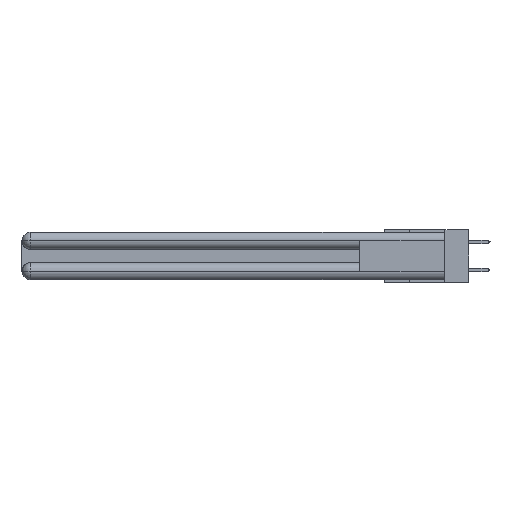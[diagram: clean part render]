
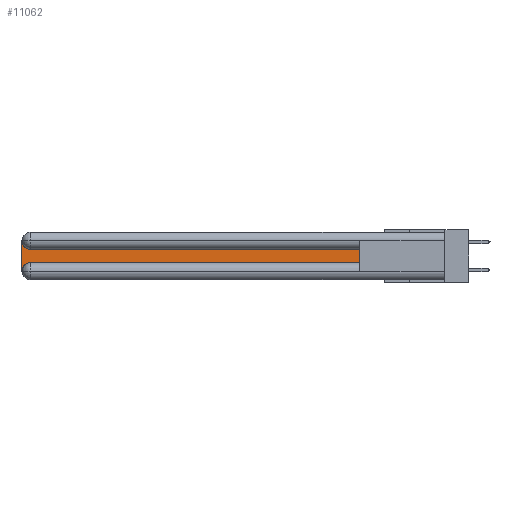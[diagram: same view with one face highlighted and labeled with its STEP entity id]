
A CAD part, left-side view. The second image highlights one B-rep face of the part: STEP entity #11062.
In plain terms, the highlighted planar face has unit normal (-1, 0, 0).
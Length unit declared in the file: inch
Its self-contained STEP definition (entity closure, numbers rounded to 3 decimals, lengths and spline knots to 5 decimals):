
#332 = LINE ( 'NONE', #25507, #10445 ) ;
#1689 = CIRCLE ( 'NONE', #16455, 0.06 ) ;
#1822 = LINE ( 'NONE', #25973, #23637 ) ;
#2093 = DIRECTION ( 'NONE',  ( 0., 0., -1. ) ) ;
#2813 = DIRECTION ( 'NONE',  ( 0., 0., -1. ) ) ;
#4516 = VECTOR ( 'NONE', #6964, 39.37008 ) ;
#6109 = EDGE_CURVE ( 'NONE', #26806, #26462, #1689, .T. ) ;
#6590 = CARTESIAN_POINT ( 'NONE',  ( 0.075, 0.6, -0.1225 ) ) ;
#6612 = EDGE_CURVE ( 'NONE', #22815, #7374, #21521, .T. ) ;
#6964 = DIRECTION ( 'NONE',  ( 0., 1., 0. ) ) ;
#7184 = DIRECTION ( 'NONE',  ( 1., 0., 0. ) ) ;
#7374 = VERTEX_POINT ( 'NONE', #23820 ) ;
#7616 = CARTESIAN_POINT ( 'NONE',  ( 0.075, 3., -0.2175 ) ) ;
#8498 = CARTESIAN_POINT ( 'NONE',  ( 0.075, 2.94, -0.2775 ) ) ;
#8811 = CARTESIAN_POINT ( 'NONE',  ( 0.075, 2.94, -0.0625 ) ) ;
#9150 = EDGE_CURVE ( 'NONE', #18460, #16581, #1822, .T. ) ;
#10445 = VECTOR ( 'NONE', #13276, 39.37008 ) ;
#11062 = ADVANCED_FACE ( 'NONE', ( #26787 ), #11156, .F. ) ;
#11156 = PLANE ( 'NONE',  #26077 ) ;
#12136 = ORIENTED_EDGE ( 'NONE', *, *, #12547, .T. ) ;
#12547 = EDGE_CURVE ( 'NONE', #7374, #18460, #332, .T. ) ;
#12778 = ORIENTED_EDGE ( 'NONE', *, *, #25248, .T. ) ;
#13134 = CARTESIAN_POINT ( 'NONE',  ( 0.075, 0.6, -0.1225 ) ) ;
#13201 = CARTESIAN_POINT ( 'NONE',  ( 0.075, 3., -0.2775 ) ) ;
#13276 = DIRECTION ( 'NONE',  ( 0., -1., 0. ) ) ;
#13728 = EDGE_CURVE ( 'NONE', #16581, #26806, #17598, .T. ) ;
#14617 = DIRECTION ( 'NONE',  ( 1., 0., 0. ) ) ;
#14838 = ORIENTED_EDGE ( 'NONE', *, *, #9150, .T. ) ;
#16455 = AXIS2_PLACEMENT_3D ( 'NONE', #8811, #23503, #23312 ) ;
#16526 = ORIENTED_EDGE ( 'NONE', *, *, #6109, .T. ) ;
#16581 = VERTEX_POINT ( 'NONE', #6590 ) ;
#17197 = ORIENTED_EDGE ( 'NONE', *, *, #13728, .T. ) ;
#17350 = DIRECTION ( 'NONE',  ( 0., 0., 1. ) ) ;
#17598 = LINE ( 'NONE', #13134, #4516 ) ;
#17881 = VECTOR ( 'NONE', #22157, 39.37008 ) ;
#18460 = VERTEX_POINT ( 'NONE', #26790 ) ;
#19855 = CARTESIAN_POINT ( 'NONE',  ( 0.075, 3., -0.0625 ) ) ;
#21521 = CIRCLE ( 'NONE', #26194, 0.06 ) ;
#22157 = DIRECTION ( 'NONE',  ( 0., 0., -1. ) ) ;
#22815 = VERTEX_POINT ( 'NONE', #13201 ) ;
#23188 = EDGE_LOOP ( 'NONE', ( #17197, #16526, #12778, #23873, #12136, #14838 ) ) ;
#23312 = DIRECTION ( 'NONE',  ( 0., 0., -1. ) ) ;
#23362 = LINE ( 'NONE', #7616, #17881 ) ;
#23503 = DIRECTION ( 'NONE',  ( 1., 0., 0. ) ) ;
#23637 = VECTOR ( 'NONE', #17350, 39.37008 ) ;
#23820 = CARTESIAN_POINT ( 'NONE',  ( 0.075, 2.94, -0.2175 ) ) ;
#23873 = ORIENTED_EDGE ( 'NONE', *, *, #6612, .T. ) ;
#24834 = CARTESIAN_POINT ( 'NONE',  ( 0.075, 2.94, -0.1225 ) ) ;
#25248 = EDGE_CURVE ( 'NONE', #26462, #22815, #23362, .T. ) ;
#25507 = CARTESIAN_POINT ( 'NONE',  ( 0.075, 0.6, -0.2175 ) ) ;
#25759 = CARTESIAN_POINT ( 'NONE',  ( 0.075, 3., -0.1225 ) ) ;
#25973 = CARTESIAN_POINT ( 'NONE',  ( 0.075, 0.6, -0.2175 ) ) ;
#26077 = AXIS2_PLACEMENT_3D ( 'NONE', #25759, #7184, #2813 ) ;
#26194 = AXIS2_PLACEMENT_3D ( 'NONE', #8498, #14617, #2093 ) ;
#26462 = VERTEX_POINT ( 'NONE', #19855 ) ;
#26787 = FACE_OUTER_BOUND ( 'NONE', #23188, .T. ) ;
#26790 = CARTESIAN_POINT ( 'NONE',  ( 0.075, 0.6, -0.2175 ) ) ;
#26806 = VERTEX_POINT ( 'NONE', #24834 ) ;
